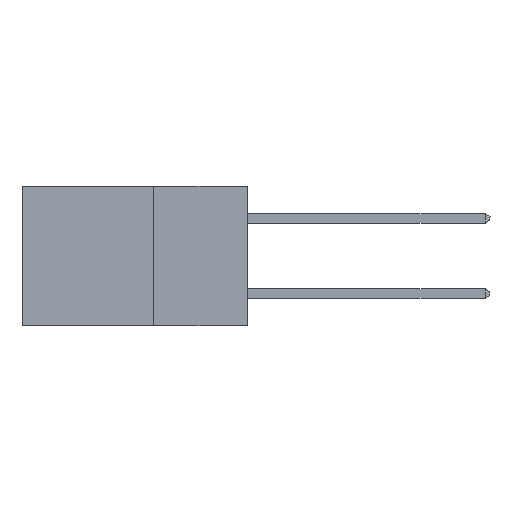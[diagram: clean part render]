
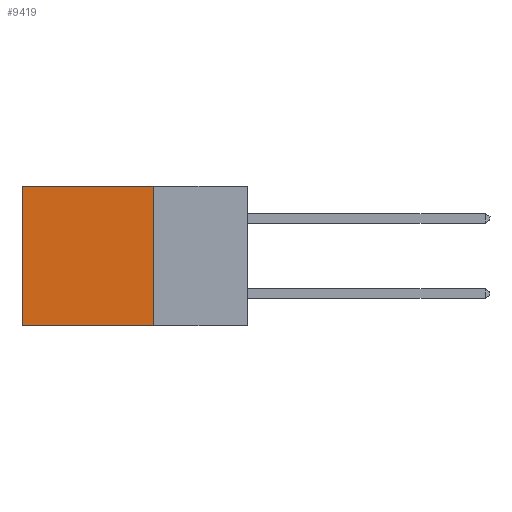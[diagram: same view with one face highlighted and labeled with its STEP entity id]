
A CAD part, left-side view. The second image highlights one B-rep face of the part: STEP entity #9419.
In plain terms, the highlighted planar face has unit normal (-1, 0, 0).
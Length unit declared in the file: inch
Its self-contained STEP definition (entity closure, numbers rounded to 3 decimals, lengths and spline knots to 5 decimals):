
#351 = CARTESIAN_POINT ( 'NONE',  ( 0.2615, 0.25, 0. ) ) ;
#653 = ORIENTED_EDGE ( 'NONE', *, *, #8085, .F. ) ;
#862 = DIRECTION ( 'NONE',  ( 0., 0., -1. ) ) ;
#1906 = FACE_OUTER_BOUND ( 'NONE', #1940, .T. ) ;
#1940 = EDGE_LOOP ( 'NONE', ( #10375, #653, #5581, #6476 ) ) ;
#2221 = DIRECTION ( 'NONE',  ( 0., 0., -1. ) ) ;
#2270 = LINE ( 'NONE', #3062, #3562 ) ;
#2612 = CARTESIAN_POINT ( 'NONE',  ( 0.2615, 0.25, -0.37 ) ) ;
#3062 = CARTESIAN_POINT ( 'NONE',  ( 0.2615, 0.6, -0.37 ) ) ;
#3489 = EDGE_CURVE ( 'NONE', #7823, #7425, #4297, .T. ) ;
#3562 = VECTOR ( 'NONE', #2221, 39.37008 ) ;
#3601 = DIRECTION ( 'NONE',  ( 0., 0., -1. ) ) ;
#3880 = CARTESIAN_POINT ( 'NONE',  ( 0.2615, 0.25, -0.37 ) ) ;
#4178 = DIRECTION ( 'NONE',  ( 0., 1., 0. ) ) ;
#4297 = LINE ( 'NONE', #2612, #7224 ) ;
#4881 = EDGE_CURVE ( 'NONE', #7823, #7503, #5328, .T. ) ;
#5279 = DIRECTION ( 'NONE',  ( 1., 0., 0. ) ) ;
#5328 = LINE ( 'NONE', #9537, #7671 ) ;
#5581 = ORIENTED_EDGE ( 'NONE', *, *, #3489, .F. ) ;
#6248 = PLANE ( 'NONE',  #9882 ) ;
#6476 = ORIENTED_EDGE ( 'NONE', *, *, #4881, .T. ) ;
#6888 = VERTEX_POINT ( 'NONE', #10104 ) ;
#7224 = VECTOR ( 'NONE', #862, 39.37008 ) ;
#7425 = VERTEX_POINT ( 'NONE', #3880 ) ;
#7469 = VECTOR ( 'NONE', #4178, 39.37008 ) ;
#7503 = VERTEX_POINT ( 'NONE', #9563 ) ;
#7671 = VECTOR ( 'NONE', #8777, 39.37008 ) ;
#7823 = VERTEX_POINT ( 'NONE', #351 ) ;
#7893 = CARTESIAN_POINT ( 'NONE',  ( 0.2615, 0.25, -0.37 ) ) ;
#8085 = EDGE_CURVE ( 'NONE', #7425, #6888, #9057, .T. ) ;
#8261 = CARTESIAN_POINT ( 'NONE',  ( 0.2615, 0.25, -0.37 ) ) ;
#8777 = DIRECTION ( 'NONE',  ( 0., 1., 0. ) ) ;
#9057 = LINE ( 'NONE', #8261, #7469 ) ;
#9419 = ADVANCED_FACE ( 'NONE', ( #1906 ), #6248, .F. ) ;
#9537 = CARTESIAN_POINT ( 'NONE',  ( 0.2615, 0.25, 0. ) ) ;
#9563 = CARTESIAN_POINT ( 'NONE',  ( 0.2615, 0.6, 0. ) ) ;
#9611 = EDGE_CURVE ( 'NONE', #7503, #6888, #2270, .T. ) ;
#9882 = AXIS2_PLACEMENT_3D ( 'NONE', #7893, #5279, #3601 ) ;
#10104 = CARTESIAN_POINT ( 'NONE',  ( 0.2615, 0.6, -0.37 ) ) ;
#10375 = ORIENTED_EDGE ( 'NONE', *, *, #9611, .T. ) ;
